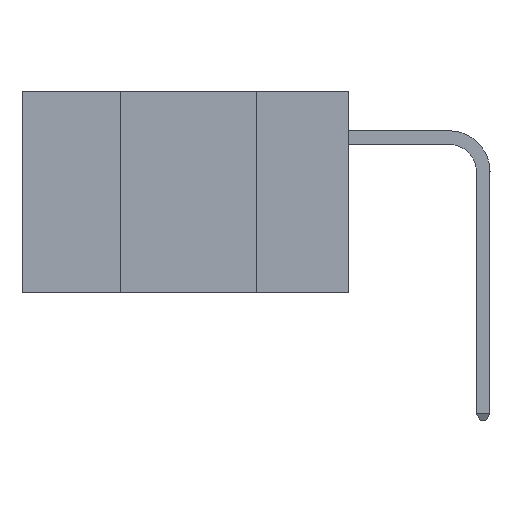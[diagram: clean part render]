
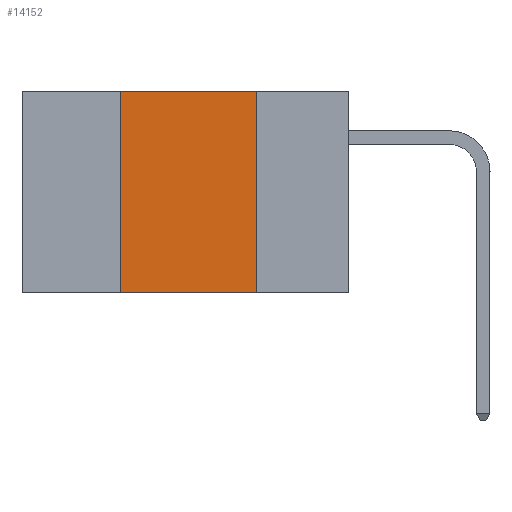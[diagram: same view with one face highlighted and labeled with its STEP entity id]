
A CAD part, left-side view. The second image highlights one B-rep face of the part: STEP entity #14152.
In plain terms, the highlighted planar face has unit normal (-1, 0, 0).
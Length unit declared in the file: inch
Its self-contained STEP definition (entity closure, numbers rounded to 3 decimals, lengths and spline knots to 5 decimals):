
#1049 = LINE ( 'NONE', #3501, #21965 ) ;
#1317 = PLANE ( 'NONE',  #3677 ) ;
#1753 = CARTESIAN_POINT ( 'NONE',  ( 0., 0.17, 0. ) ) ;
#1916 = DIRECTION ( 'NONE',  ( 0., -1., 0. ) ) ;
#3196 = EDGE_LOOP ( 'NONE', ( #11854, #12621, #25057, #15275 ) ) ;
#3501 = CARTESIAN_POINT ( 'NONE',  ( 0., 0.17, 0. ) ) ;
#3533 = CARTESIAN_POINT ( 'NONE',  ( 0., 0.42, 0. ) ) ;
#3677 = AXIS2_PLACEMENT_3D ( 'NONE', #15482, #17533, #5361 ) ;
#3750 = EDGE_CURVE ( 'NONE', #6978, #11851, #1049, .T. ) ;
#4399 = LINE ( 'NONE', #3533, #15195 ) ;
#5361 = DIRECTION ( 'NONE',  ( 0., 0., -1. ) ) ;
#5451 = FACE_OUTER_BOUND ( 'NONE', #3196, .T. ) ;
#5471 = DIRECTION ( 'NONE',  ( 0., 0., -1. ) ) ;
#6978 = VERTEX_POINT ( 'NONE', #1753 ) ;
#7017 = EDGE_CURVE ( 'NONE', #16414, #6978, #26185, .T. ) ;
#8023 = CARTESIAN_POINT ( 'NONE',  ( 0., 0.42, 0. ) ) ;
#8757 = LINE ( 'NONE', #26083, #14797 ) ;
#10205 = CARTESIAN_POINT ( 'NONE',  ( 0., 0.42, -0.37 ) ) ;
#11851 = VERTEX_POINT ( 'NONE', #18187 ) ;
#11854 = ORIENTED_EDGE ( 'NONE', *, *, #3750, .F. ) ;
#11893 = CARTESIAN_POINT ( 'NONE',  ( 0., 0.6, 0. ) ) ;
#12621 = ORIENTED_EDGE ( 'NONE', *, *, #7017, .F. ) ;
#14152 = ADVANCED_FACE ( 'NONE', ( #5451 ), #1317, .F. ) ;
#14797 = VECTOR ( 'NONE', #16000, 39.37008 ) ;
#15195 = VECTOR ( 'NONE', #17760, 39.37008 ) ;
#15275 = ORIENTED_EDGE ( 'NONE', *, *, #18296, .T. ) ;
#15482 = CARTESIAN_POINT ( 'NONE',  ( 0., 0.6, 0. ) ) ;
#15565 = EDGE_CURVE ( 'NONE', #22876, #16414, #4399, .T. ) ;
#16000 = DIRECTION ( 'NONE',  ( 0., -1., 0. ) ) ;
#16414 = VERTEX_POINT ( 'NONE', #8023 ) ;
#17533 = DIRECTION ( 'NONE',  ( 1., 0., 0. ) ) ;
#17760 = DIRECTION ( 'NONE',  ( 0., 0., 1. ) ) ;
#18187 = CARTESIAN_POINT ( 'NONE',  ( 0., 0.17, -0.37 ) ) ;
#18296 = EDGE_CURVE ( 'NONE', #22876, #11851, #8757, .T. ) ;
#20179 = VECTOR ( 'NONE', #1916, 39.37008 ) ;
#21965 = VECTOR ( 'NONE', #5471, 39.37008 ) ;
#22876 = VERTEX_POINT ( 'NONE', #10205 ) ;
#25057 = ORIENTED_EDGE ( 'NONE', *, *, #15565, .F. ) ;
#26083 = CARTESIAN_POINT ( 'NONE',  ( 0., 0.6, -0.37 ) ) ;
#26185 = LINE ( 'NONE', #11893, #20179 ) ;
